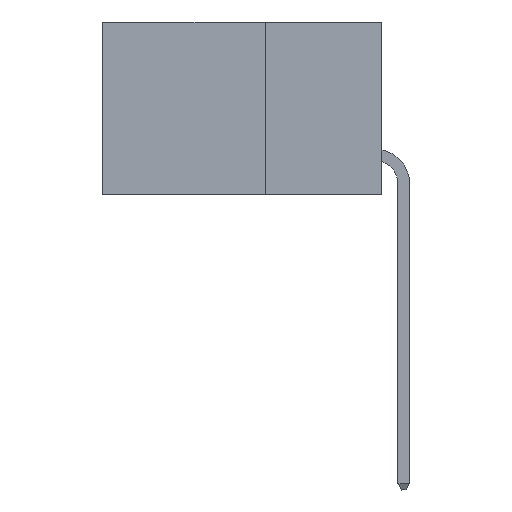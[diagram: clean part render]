
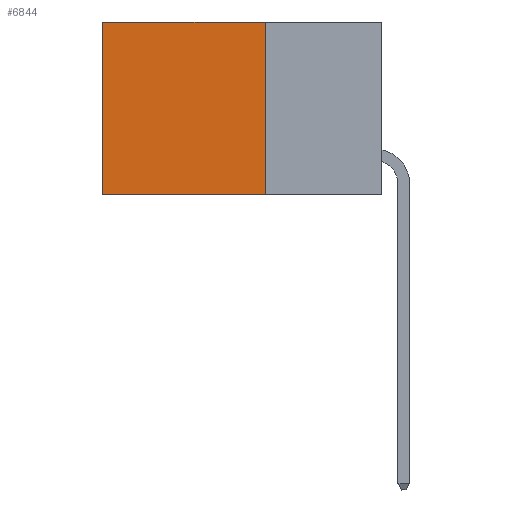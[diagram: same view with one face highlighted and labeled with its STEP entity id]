
A CAD part, left-side view. The second image highlights one B-rep face of the part: STEP entity #6844.
In plain terms, the highlighted planar face has unit normal (-1, 0, 0).
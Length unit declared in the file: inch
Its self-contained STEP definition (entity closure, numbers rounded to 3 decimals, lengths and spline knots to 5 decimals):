
#302 = CARTESIAN_POINT ( 'NONE',  ( 0.2875, 0.25, -0.37 ) ) ;
#541 = ORIENTED_EDGE ( 'NONE', *, *, #9503, .F. ) ;
#812 = LINE ( 'NONE', #10617, #16781 ) ;
#1737 = DIRECTION ( 'NONE',  ( 0., 0., -1. ) ) ;
#4651 = ORIENTED_EDGE ( 'NONE', *, *, #13308, .T. ) ;
#5064 = DIRECTION ( 'NONE',  ( 0., 1., 0. ) ) ;
#6814 = VERTEX_POINT ( 'NONE', #21545 ) ;
#6844 = ADVANCED_FACE ( 'NONE', ( #15546 ), #11070, .F. ) ;
#7527 = VECTOR ( 'NONE', #13867, 39.37008 ) ;
#7572 = DIRECTION ( 'NONE',  ( 1., 0., 0. ) ) ;
#8187 = LINE ( 'NONE', #9254, #7527 ) ;
#9222 = CARTESIAN_POINT ( 'NONE',  ( 0.2875, 0.25, 0. ) ) ;
#9254 = CARTESIAN_POINT ( 'NONE',  ( 0.2875, 0.6, 0. ) ) ;
#9503 = EDGE_CURVE ( 'NONE', #18085, #11420, #17348, .T. ) ;
#9911 = CARTESIAN_POINT ( 'NONE',  ( 0.2875, 0.25, -0.37 ) ) ;
#10617 = CARTESIAN_POINT ( 'NONE',  ( 0.2875, 0.25, 0. ) ) ;
#11070 = PLANE ( 'NONE',  #25807 ) ;
#11420 = VERTEX_POINT ( 'NONE', #20695 ) ;
#11711 = VECTOR ( 'NONE', #21348, 39.37008 ) ;
#13308 = EDGE_CURVE ( 'NONE', #14269, #11420, #8187, .T. ) ;
#13679 = ORIENTED_EDGE ( 'NONE', *, *, #22033, .T. ) ;
#13867 = DIRECTION ( 'NONE',  ( 0., 0., -1. ) ) ;
#14269 = VERTEX_POINT ( 'NONE', #19138 ) ;
#15546 = FACE_OUTER_BOUND ( 'NONE', #16401, .T. ) ;
#16401 = EDGE_LOOP ( 'NONE', ( #4651, #541, #25766, #13679 ) ) ;
#16431 = VECTOR ( 'NONE', #5064, 39.37008 ) ;
#16781 = VECTOR ( 'NONE', #1737, 39.37008 ) ;
#17348 = LINE ( 'NONE', #302, #11711 ) ;
#18085 = VERTEX_POINT ( 'NONE', #9911 ) ;
#18382 = CARTESIAN_POINT ( 'NONE',  ( 0.2875, 0.25, 0. ) ) ;
#19138 = CARTESIAN_POINT ( 'NONE',  ( 0.2875, 0.6, 0. ) ) ;
#20695 = CARTESIAN_POINT ( 'NONE',  ( 0.2875, 0.6, -0.37 ) ) ;
#21348 = DIRECTION ( 'NONE',  ( 0., 1., 0. ) ) ;
#21545 = CARTESIAN_POINT ( 'NONE',  ( 0.2875, 0.25, 0. ) ) ;
#21887 = EDGE_CURVE ( 'NONE', #6814, #18085, #812, .T. ) ;
#22033 = EDGE_CURVE ( 'NONE', #6814, #14269, #27299, .T. ) ;
#22550 = DIRECTION ( 'NONE',  ( 0., 0., -1. ) ) ;
#25766 = ORIENTED_EDGE ( 'NONE', *, *, #21887, .F. ) ;
#25807 = AXIS2_PLACEMENT_3D ( 'NONE', #18382, #7572, #22550 ) ;
#27299 = LINE ( 'NONE', #9222, #16431 ) ;
